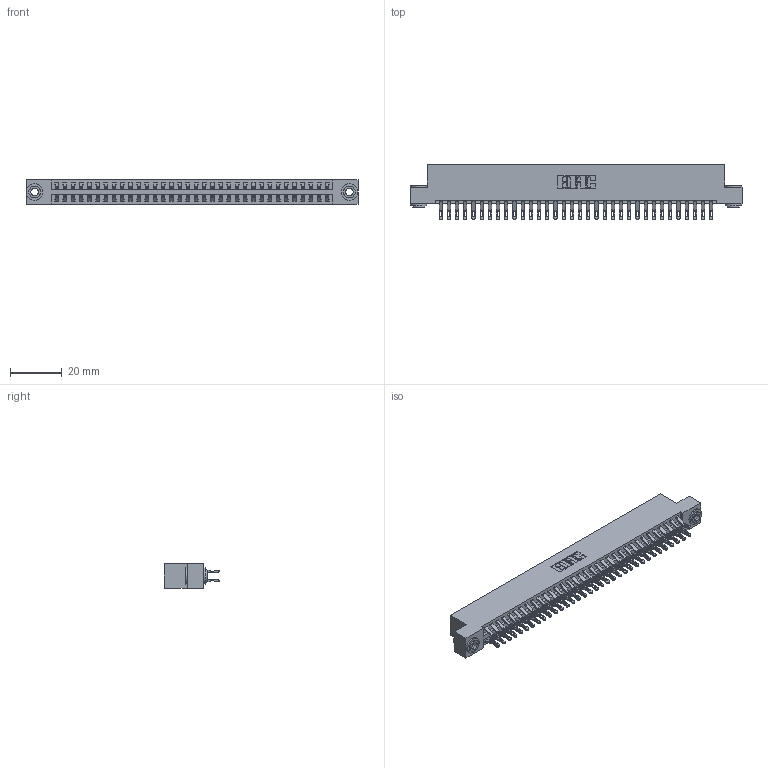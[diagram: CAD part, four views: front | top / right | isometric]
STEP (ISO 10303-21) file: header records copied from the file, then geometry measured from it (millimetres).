
FILE_DESCRIPTION (( 'STEP AP203' ), '1' );
FILE_NAME ('346-068-555-203.STEP', '2022-05-24T19:37:56', ( '' ), ( '' ), 'SwSTEP 2.0', 'SolidWorks 2020', '' );
FILE_SCHEMA (( 'CONFIG_CONTROL_DESIGN' ));
Length unit declared in the file: inch
Products named in the file (4): 345-292-001_555 Tail; 345-250-002_345-250-002-102; 346-068-555-203; 346 Part_Flush Mounting Lugs - 0.156 Dia-TH
Assembly tree (71 placements, depth 2):
  346-068-555-203
    346 Part_Flush Mounting Lugs - 0.156 Dia-TH
    345-292-001_555 Tail  x68
    345-250-002_345-250-002-102  x2
Bounding box: 128.52 x 21.46 x 9.4 mm (x, y, z)
Volume: 12669.1 mm3; surface area: 18240.6 mm2
Topology: 71 solids, 71 shells, 4118 faces, 12885 edges, 8586 vertices
Faces by surface type: plane 2344, cylinder 1766, cone 8
Entity records: 24658 total; most frequent: CARTESIAN_POINT 4091, ORIENTED_EDGE 3986, DIRECTION 3655, EDGE_CURVE 1993, VECTOR 1681, LINE 1681, VERTEX_POINT 1326, AXIS2_PLACEMENT_3D 987
